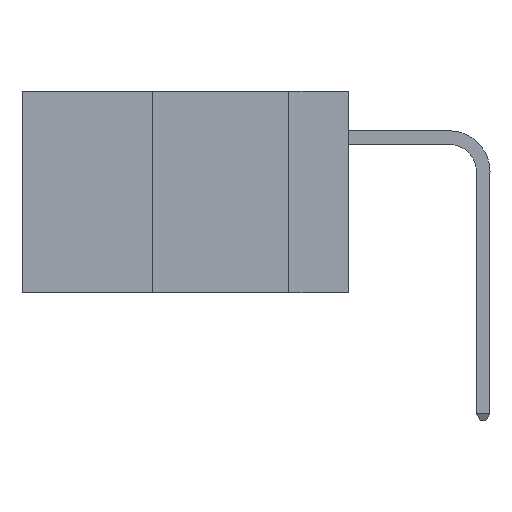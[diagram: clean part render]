
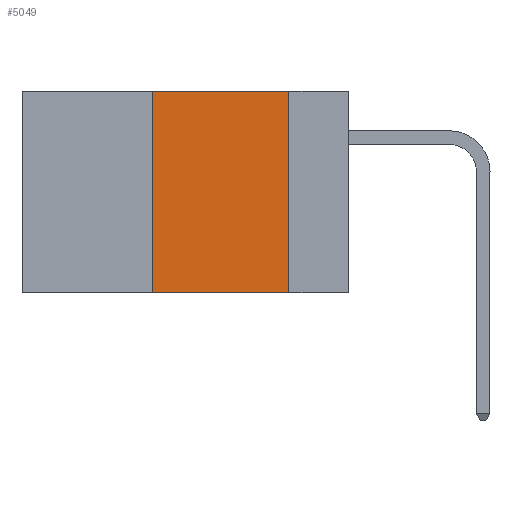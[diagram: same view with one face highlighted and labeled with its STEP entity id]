
A CAD part, left-side view. The second image highlights one B-rep face of the part: STEP entity #5049.
In plain terms, the highlighted planar face has unit normal (-1, 0, 0).
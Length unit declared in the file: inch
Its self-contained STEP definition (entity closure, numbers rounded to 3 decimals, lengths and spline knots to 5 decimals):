
#581 = CARTESIAN_POINT ( 'NONE',  ( 0., 0.36, -0.37 ) ) ;
#665 = ORIENTED_EDGE ( 'NONE', *, *, #8408, .T. ) ;
#1043 = EDGE_CURVE ( 'NONE', #7635, #4473, #4871, .T. ) ;
#1712 = LINE ( 'NONE', #5484, #9208 ) ;
#1956 = VERTEX_POINT ( 'NONE', #581 ) ;
#2012 = VECTOR ( 'NONE', #9293, 39.37008 ) ;
#2041 = CARTESIAN_POINT ( 'NONE',  ( 0., 0.6, 0. ) ) ;
#2315 = LINE ( 'NONE', #12196, #2012 ) ;
#3104 = ORIENTED_EDGE ( 'NONE', *, *, #8461, .F. ) ;
#4009 = CARTESIAN_POINT ( 'NONE',  ( 0., 0.6, 0. ) ) ;
#4039 = CARTESIAN_POINT ( 'NONE',  ( 0., 0.11, 0. ) ) ;
#4473 = VERTEX_POINT ( 'NONE', #7001 ) ;
#4871 = LINE ( 'NONE', #10096, #6582 ) ;
#5043 = DIRECTION ( 'NONE',  ( 0., 0., -1. ) ) ;
#5049 = ADVANCED_FACE ( 'NONE', ( #8809 ), #8941, .F. ) ;
#5484 = CARTESIAN_POINT ( 'NONE',  ( 0., 0.36, 0. ) ) ;
#5666 = LINE ( 'NONE', #2041, #7983 ) ;
#6166 = DIRECTION ( 'NONE',  ( 0., 0., -1. ) ) ;
#6477 = VERTEX_POINT ( 'NONE', #10152 ) ;
#6582 = VECTOR ( 'NONE', #6166, 39.37008 ) ;
#7001 = CARTESIAN_POINT ( 'NONE',  ( 0., 0.11, -0.37 ) ) ;
#7567 = ORIENTED_EDGE ( 'NONE', *, *, #10090, .F. ) ;
#7635 = VERTEX_POINT ( 'NONE', #4039 ) ;
#7983 = VECTOR ( 'NONE', #9879, 39.37008 ) ;
#8408 = EDGE_CURVE ( 'NONE', #1956, #4473, #2315, .T. ) ;
#8461 = EDGE_CURVE ( 'NONE', #1956, #6477, #1712, .T. ) ;
#8809 = FACE_OUTER_BOUND ( 'NONE', #10209, .T. ) ;
#8941 = PLANE ( 'NONE',  #10826 ) ;
#9208 = VECTOR ( 'NONE', #12281, 39.37008 ) ;
#9293 = DIRECTION ( 'NONE',  ( 0., -1., 0. ) ) ;
#9879 = DIRECTION ( 'NONE',  ( 0., -1., 0. ) ) ;
#10090 = EDGE_CURVE ( 'NONE', #6477, #7635, #5666, .T. ) ;
#10096 = CARTESIAN_POINT ( 'NONE',  ( 0., 0.11, 0. ) ) ;
#10152 = CARTESIAN_POINT ( 'NONE',  ( 0., 0.36, 0. ) ) ;
#10209 = EDGE_LOOP ( 'NONE', ( #11946, #7567, #3104, #665 ) ) ;
#10826 = AXIS2_PLACEMENT_3D ( 'NONE', #4009, #10896, #5043 ) ;
#10896 = DIRECTION ( 'NONE',  ( 1., 0., 0. ) ) ;
#11946 = ORIENTED_EDGE ( 'NONE', *, *, #1043, .F. ) ;
#12196 = CARTESIAN_POINT ( 'NONE',  ( 0., 0.6, -0.37 ) ) ;
#12281 = DIRECTION ( 'NONE',  ( 0., 0., 1. ) ) ;
